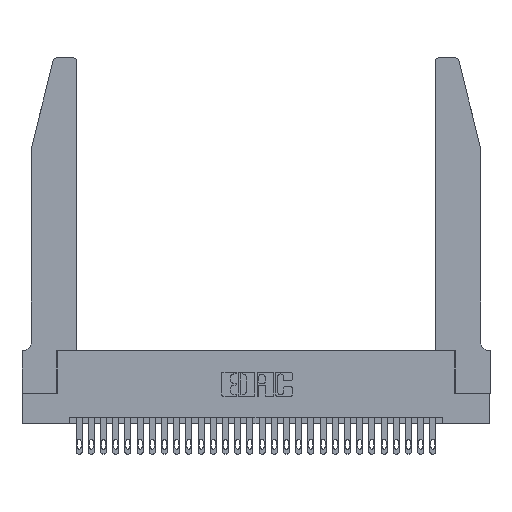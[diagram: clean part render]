
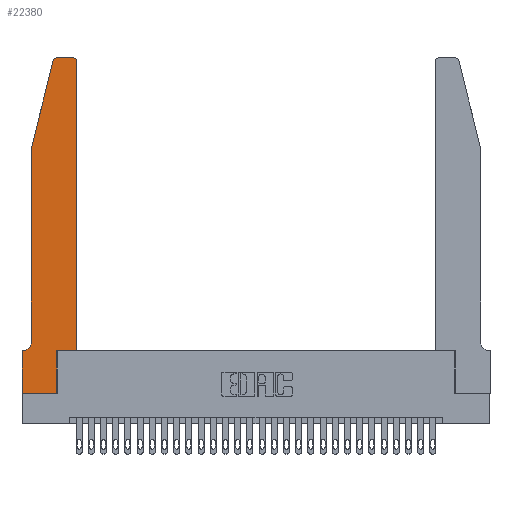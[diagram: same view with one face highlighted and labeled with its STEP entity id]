
A CAD part, top view. The second image highlights one B-rep face of the part: STEP entity #22380.
In plain terms, the highlighted planar face has unit normal (0, 0, 1).
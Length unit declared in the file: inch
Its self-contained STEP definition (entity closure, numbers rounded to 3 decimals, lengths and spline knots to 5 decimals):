
#782 = CIRCLE ( 'NONE', #17721, 0.07 ) ;
#819 = VERTEX_POINT ( 'NONE', #22696 ) ;
#1336 = ORIENTED_EDGE ( 'NONE', *, *, #16815, .T. ) ;
#1620 = VECTOR ( 'NONE', #10068, 39.37008 ) ;
#1765 = DIRECTION ( 'NONE',  ( 0., 0., -1. ) ) ;
#2299 = ORIENTED_EDGE ( 'NONE', *, *, #7768, .T. ) ;
#2523 = VECTOR ( 'NONE', #11944, 39.37008 ) ;
#3090 = CARTESIAN_POINT ( 'NONE',  ( 0.4505, 0.35, 0.37 ) ) ;
#3396 = EDGE_CURVE ( 'NONE', #14578, #26228, #19353, .T. ) ;
#3548 = VECTOR ( 'NONE', #17703, 39.37008 ) ;
#3746 = ORIENTED_EDGE ( 'NONE', *, *, #12257, .T. ) ;
#3895 = CARTESIAN_POINT ( 'NONE',  ( 0., 0.35, 0.37 ) ) ;
#3920 = CARTESIAN_POINT ( 'NONE',  ( 0.284, 2.75, 0.37 ) ) ;
#4548 = VECTOR ( 'NONE', #9349, 39.37008 ) ;
#4934 = EDGE_CURVE ( 'NONE', #819, #5278, #10678, .T. ) ;
#5009 = CARTESIAN_POINT ( 'NONE',  ( 0., 0.35, 0.37 ) ) ;
#5031 = CARTESIAN_POINT ( 'NONE',  ( 0.0755, 0.42, 0.37 ) ) ;
#5067 = DIRECTION ( 'NONE',  ( 1., 0., 0. ) ) ;
#5278 = VERTEX_POINT ( 'NONE', #9522 ) ;
#5364 = CARTESIAN_POINT ( 'NONE',  ( 0.25487, 2.72718, 0.37 ) ) ;
#5416 = CARTESIAN_POINT ( 'NONE',  ( 0.0755, 2., 0.37 ) ) ;
#6048 = CARTESIAN_POINT ( 'NONE',  ( 0.0055, 0.35, 0.37 ) ) ;
#6781 = AXIS2_PLACEMENT_3D ( 'NONE', #5009, #20885, #11812 ) ;
#6936 = FACE_OUTER_BOUND ( 'NONE', #7715, .T. ) ;
#7205 = CARTESIAN_POINT ( 'NONE',  ( 0.284, 2.72, 0.37 ) ) ;
#7549 = PLANE ( 'NONE',  #6781 ) ;
#7715 = EDGE_LOOP ( 'NONE', ( #22734, #17681, #2299, #12501, #3746, #18475, #14438, #1336, #13892, #19700, #8694, #8429 ) ) ;
#7768 = EDGE_CURVE ( 'NONE', #21668, #28964, #26797, .T. ) ;
#7843 = DIRECTION ( 'NONE',  ( 1., 0., 0. ) ) ;
#8293 = DIRECTION ( 'NONE',  ( -1., 0., 0. ) ) ;
#8429 = ORIENTED_EDGE ( 'NONE', *, *, #18617, .T. ) ;
#8501 = CARTESIAN_POINT ( 'NONE',  ( 0.0055, 0.42, 0.37 ) ) ;
#8652 = EDGE_CURVE ( 'NONE', #28647, #11904, #28154, .T. ) ;
#8694 = ORIENTED_EDGE ( 'NONE', *, *, #4934, .T. ) ;
#9043 = EDGE_CURVE ( 'NONE', #28964, #27844, #22343, .T. ) ;
#9238 = CARTESIAN_POINT ( 'NONE',  ( 0.4205, 2.75, 0.37 ) ) ;
#9349 = DIRECTION ( 'NONE',  ( 1., 0., 0. ) ) ;
#9411 = CARTESIAN_POINT ( 'NONE',  ( 0.2865, 0., 0.37 ) ) ;
#9522 = CARTESIAN_POINT ( 'NONE',  ( 0.4505, 2.72, 0.37 ) ) ;
#9554 = CARTESIAN_POINT ( 'NONE',  ( 0.2605, 2.75, 0.37 ) ) ;
#10068 = DIRECTION ( 'NONE',  ( -0.239, -0.971, 0. ) ) ;
#10188 = CARTESIAN_POINT ( 'NONE',  ( 0.2865, 0.35, 0.37 ) ) ;
#10282 = LINE ( 'NONE', #22930, #11379 ) ;
#10678 = LINE ( 'NONE', #3090, #21399 ) ;
#10838 = DIRECTION ( 'NONE',  ( 0., 0., 1. ) ) ;
#11379 = VECTOR ( 'NONE', #15389, 39.37008 ) ;
#11575 = CIRCLE ( 'NONE', #19192, 0.03 ) ;
#11812 = DIRECTION ( 'NONE',  ( 1., 0., 0. ) ) ;
#11904 = VERTEX_POINT ( 'NONE', #23531 ) ;
#11944 = DIRECTION ( 'NONE',  ( -1., 0., 0. ) ) ;
#12056 = DIRECTION ( 'NONE',  ( 0., 0., 1. ) ) ;
#12257 = EDGE_CURVE ( 'NONE', #27844, #12602, #782, .T. ) ;
#12501 = ORIENTED_EDGE ( 'NONE', *, *, #9043, .T. ) ;
#12602 = VERTEX_POINT ( 'NONE', #6048 ) ;
#12656 = VECTOR ( 'NONE', #26512, 39.37008 ) ;
#12965 = CARTESIAN_POINT ( 'NONE',  ( 0.4205, 2.72, 0.37 ) ) ;
#12972 = CIRCLE ( 'NONE', #27817, 0.03 ) ;
#13892 = ORIENTED_EDGE ( 'NONE', *, *, #3396, .T. ) ;
#14438 = ORIENTED_EDGE ( 'NONE', *, *, #8652, .T. ) ;
#14578 = VERTEX_POINT ( 'NONE', #9411 ) ;
#14730 = CARTESIAN_POINT ( 'NONE',  ( 0.4505, 0.35, 0.37 ) ) ;
#14972 = EDGE_CURVE ( 'NONE', #18832, #21668, #12972, .T. ) ;
#15141 = VECTOR ( 'NONE', #26110, 39.37008 ) ;
#15389 = DIRECTION ( 'NONE',  ( -1., 0., 0. ) ) ;
#16815 = EDGE_CURVE ( 'NONE', #11904, #14578, #28662, .T. ) ;
#17681 = ORIENTED_EDGE ( 'NONE', *, *, #14972, .T. ) ;
#17703 = DIRECTION ( 'NONE',  ( 0., 1., 0. ) ) ;
#17721 = AXIS2_PLACEMENT_3D ( 'NONE', #8501, #1765, #8293 ) ;
#18142 = EDGE_CURVE ( 'NONE', #12602, #28647, #10282, .T. ) ;
#18475 = ORIENTED_EDGE ( 'NONE', *, *, #18142, .T. ) ;
#18617 = EDGE_CURVE ( 'NONE', #5278, #24018, #11575, .T. ) ;
#18832 = VERTEX_POINT ( 'NONE', #3920 ) ;
#19192 = AXIS2_PLACEMENT_3D ( 'NONE', #12965, #10838, #22153 ) ;
#19353 = LINE ( 'NONE', #19831, #3548 ) ;
#19700 = ORIENTED_EDGE ( 'NONE', *, *, #24922, .T. ) ;
#19831 = CARTESIAN_POINT ( 'NONE',  ( 0.2865, 0.35, 0.37 ) ) ;
#20885 = DIRECTION ( 'NONE',  ( 0., 0., 1. ) ) ;
#21399 = VECTOR ( 'NONE', #23552, 39.37008 ) ;
#21668 = VERTEX_POINT ( 'NONE', #5364 ) ;
#22153 = DIRECTION ( 'NONE',  ( 1., 0., 0. ) ) ;
#22343 = LINE ( 'NONE', #28840, #12656 ) ;
#22380 = ADVANCED_FACE ( 'NONE', ( #6936 ), #7549, .T. ) ;
#22696 = CARTESIAN_POINT ( 'NONE',  ( 0.4505, 0.35, 0.37 ) ) ;
#22734 = ORIENTED_EDGE ( 'NONE', *, *, #27103, .T. ) ;
#22930 = CARTESIAN_POINT ( 'NONE',  ( 0.0755, 0.35, 0.37 ) ) ;
#23142 = CARTESIAN_POINT ( 'NONE',  ( 0., 0., 0.37 ) ) ;
#23531 = CARTESIAN_POINT ( 'NONE',  ( 0., 0., 0.37 ) ) ;
#23552 = DIRECTION ( 'NONE',  ( 0., 1., 0. ) ) ;
#24018 = VERTEX_POINT ( 'NONE', #9238 ) ;
#24922 = EDGE_CURVE ( 'NONE', #26228, #819, #25142, .T. ) ;
#25142 = LINE ( 'NONE', #14730, #28382 ) ;
#25494 = CARTESIAN_POINT ( 'NONE',  ( 0.0755, 2., 0.37 ) ) ;
#26110 = DIRECTION ( 'NONE',  ( 0., -1., 0. ) ) ;
#26228 = VERTEX_POINT ( 'NONE', #10188 ) ;
#26242 = LINE ( 'NONE', #9554, #2523 ) ;
#26512 = DIRECTION ( 'NONE',  ( 0., -1., 0. ) ) ;
#26797 = LINE ( 'NONE', #5416, #1620 ) ;
#27103 = EDGE_CURVE ( 'NONE', #24018, #18832, #26242, .T. ) ;
#27817 = AXIS2_PLACEMENT_3D ( 'NONE', #7205, #12056, #5067 ) ;
#27844 = VERTEX_POINT ( 'NONE', #5031 ) ;
#28154 = LINE ( 'NONE', #28556, #15141 ) ;
#28382 = VECTOR ( 'NONE', #7843, 39.37008 ) ;
#28556 = CARTESIAN_POINT ( 'NONE',  ( 0., 0., 0.37 ) ) ;
#28647 = VERTEX_POINT ( 'NONE', #3895 ) ;
#28662 = LINE ( 'NONE', #23142, #4548 ) ;
#28840 = CARTESIAN_POINT ( 'NONE',  ( 0.0755, 2., 0.37 ) ) ;
#28964 = VERTEX_POINT ( 'NONE', #25494 ) ;
